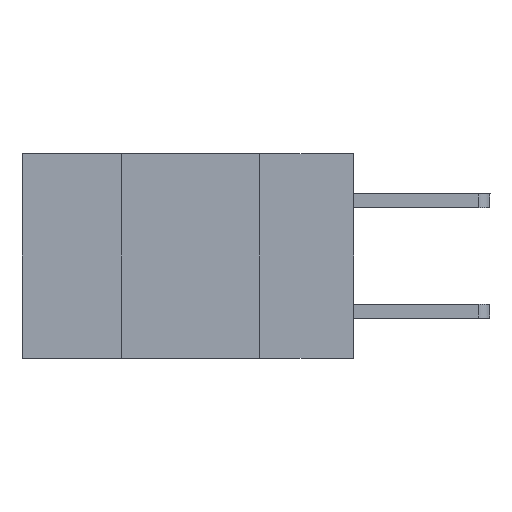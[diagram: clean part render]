
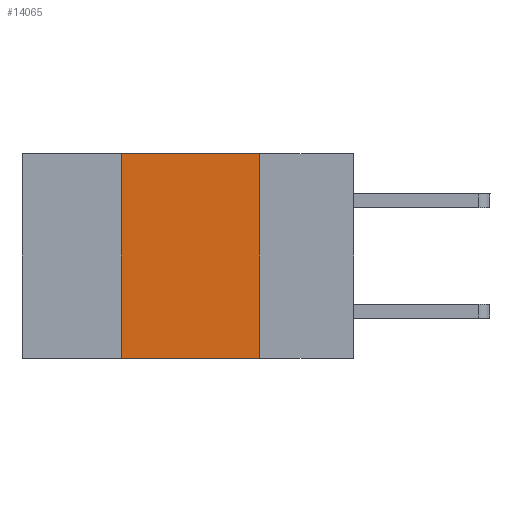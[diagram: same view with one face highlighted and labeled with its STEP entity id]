
A CAD part, left-side view. The second image highlights one B-rep face of the part: STEP entity #14065.
In plain terms, the highlighted planar face has unit normal (-1, 0, 0).
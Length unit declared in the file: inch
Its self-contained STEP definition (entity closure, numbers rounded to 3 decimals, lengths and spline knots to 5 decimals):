
#484 = ORIENTED_EDGE ( 'NONE', *, *, #4379, .T. ) ;
#986 = ORIENTED_EDGE ( 'NONE', *, *, #5232, .F. ) ;
#1122 = PLANE ( 'NONE',  #6909 ) ;
#1622 = CARTESIAN_POINT ( 'NONE',  ( 0., 0.42, 0. ) ) ;
#1824 = VERTEX_POINT ( 'NONE', #11268 ) ;
#2180 = VERTEX_POINT ( 'NONE', #5359 ) ;
#2193 = CARTESIAN_POINT ( 'NONE',  ( 0., 0.42, 0. ) ) ;
#3312 = VECTOR ( 'NONE', #15013, 39.37008 ) ;
#3483 = DIRECTION ( 'NONE',  ( 1., 0., 0. ) ) ;
#3625 = LINE ( 'NONE', #14629, #11625 ) ;
#3941 = ORIENTED_EDGE ( 'NONE', *, *, #11034, .F. ) ;
#4379 = EDGE_CURVE ( 'NONE', #2180, #1824, #9646, .T. ) ;
#4575 = ORIENTED_EDGE ( 'NONE', *, *, #12560, .F. ) ;
#5232 = EDGE_CURVE ( 'NONE', #14417, #13368, #6600, .T. ) ;
#5359 = CARTESIAN_POINT ( 'NONE',  ( 0., 0.42, -0.37 ) ) ;
#5406 = CARTESIAN_POINT ( 'NONE',  ( 0., 0.6, 0. ) ) ;
#5659 = DIRECTION ( 'NONE',  ( 0., 0., -1. ) ) ;
#5984 = EDGE_LOOP ( 'NONE', ( #4575, #986, #3941, #484 ) ) ;
#6600 = LINE ( 'NONE', #5406, #7158 ) ;
#6909 = AXIS2_PLACEMENT_3D ( 'NONE', #15282, #3483, #5659 ) ;
#7158 = VECTOR ( 'NONE', #9099, 39.37008 ) ;
#7428 = DIRECTION ( 'NONE',  ( 0., 0., -1. ) ) ;
#8109 = CARTESIAN_POINT ( 'NONE',  ( 0., 0.6, -0.37 ) ) ;
#9099 = DIRECTION ( 'NONE',  ( 0., -1., 0. ) ) ;
#9490 = DIRECTION ( 'NONE',  ( 0., 0., 1. ) ) ;
#9646 = LINE ( 'NONE', #8109, #3312 ) ;
#10620 = VECTOR ( 'NONE', #9490, 39.37008 ) ;
#11034 = EDGE_CURVE ( 'NONE', #2180, #14417, #14682, .T. ) ;
#11268 = CARTESIAN_POINT ( 'NONE',  ( 0., 0.17, -0.37 ) ) ;
#11625 = VECTOR ( 'NONE', #7428, 39.37008 ) ;
#12560 = EDGE_CURVE ( 'NONE', #13368, #1824, #3625, .T. ) ;
#12880 = FACE_OUTER_BOUND ( 'NONE', #5984, .T. ) ;
#13368 = VERTEX_POINT ( 'NONE', #14313 ) ;
#14065 = ADVANCED_FACE ( 'NONE', ( #12880 ), #1122, .F. ) ;
#14313 = CARTESIAN_POINT ( 'NONE',  ( 0., 0.17, 0. ) ) ;
#14417 = VERTEX_POINT ( 'NONE', #1622 ) ;
#14629 = CARTESIAN_POINT ( 'NONE',  ( 0., 0.17, 0. ) ) ;
#14682 = LINE ( 'NONE', #2193, #10620 ) ;
#15013 = DIRECTION ( 'NONE',  ( 0., -1., 0. ) ) ;
#15282 = CARTESIAN_POINT ( 'NONE',  ( 0., 0.6, 0. ) ) ;
